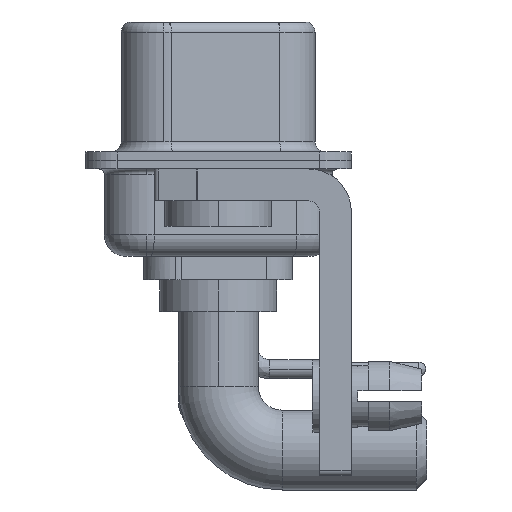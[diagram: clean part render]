
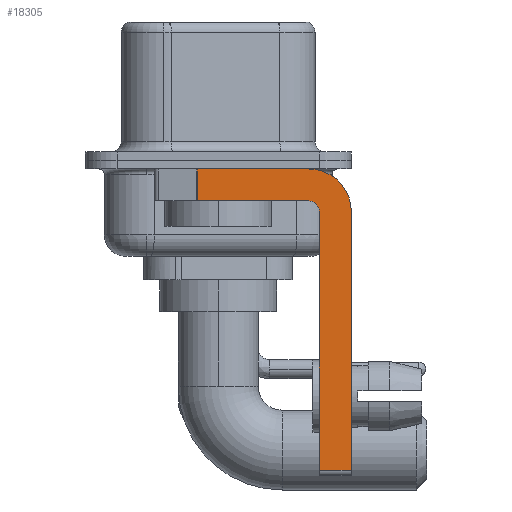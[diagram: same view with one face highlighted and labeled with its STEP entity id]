
A CAD part, left-side view. The second image highlights one B-rep face of the part: STEP entity #18305.
In plain terms, the highlighted planar face has unit normal (-1, 0, 0).
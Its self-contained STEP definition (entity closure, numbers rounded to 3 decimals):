
#687 = DIRECTION ( 'NONE',  ( 0., 0., 1. ) ) ;
#978 = CARTESIAN_POINT ( 'NONE',  ( -2.9, -4.25, -1.9 ) ) ;
#1161 = DIRECTION ( 'NONE',  ( 0., 0., -1. ) ) ;
#1473 = DIRECTION ( 'NONE',  ( 1., 0., 0. ) ) ;
#2070 = VERTEX_POINT ( 'NONE', #21945 ) ;
#2636 = CIRCLE ( 'NONE', #18275, 0.5 ) ;
#3033 = DIRECTION ( 'NONE',  ( 0., 0., 1. ) ) ;
#4359 = CARTESIAN_POINT ( 'NONE',  ( -2.9, -6.25, -2.4 ) ) ;
#4758 = VERTEX_POINT ( 'NONE', #16413 ) ;
#4934 = EDGE_CURVE ( 'NONE', #12364, #19871, #8243, .T. ) ;
#4981 = EDGE_LOOP ( 'NONE', ( #13253, #11088, #13358, #8289, #28068, #10919, #26692, #12249 ) ) ;
#5983 = CARTESIAN_POINT ( 'NONE',  ( -2.9, -4.25, -2.4 ) ) ;
#6004 = CARTESIAN_POINT ( 'NONE',  ( -2.9, -4.25, -1.9 ) ) ;
#7855 = EDGE_CURVE ( 'NONE', #4758, #14268, #2636, .T. ) ;
#7875 = CARTESIAN_POINT ( 'NONE',  ( -2.9, -4.25, -2.4 ) ) ;
#8243 = LINE ( 'NONE', #4359, #12987 ) ;
#8289 = ORIENTED_EDGE ( 'NONE', *, *, #7855, .F. ) ;
#8372 = DIRECTION ( 'NONE',  ( 1., 0., 0. ) ) ;
#8873 = CARTESIAN_POINT ( 'NONE',  ( -2.9, 3., -0.4 ) ) ;
#8938 = LINE ( 'NONE', #16047, #11588 ) ;
#10384 = VERTEX_POINT ( 'NONE', #18483 ) ;
#10616 = DIRECTION ( 'NONE',  ( 0., 0., -1. ) ) ;
#10919 = ORIENTED_EDGE ( 'NONE', *, *, #14473, .T. ) ;
#11088 = ORIENTED_EDGE ( 'NONE', *, *, #21189, .T. ) ;
#11556 = CARTESIAN_POINT ( 'NONE',  ( -2.9, -6.25, -14.55 ) ) ;
#11588 = VECTOR ( 'NONE', #25247, 1000. ) ;
#11960 = LINE ( 'NONE', #13356, #14738 ) ;
#12249 = ORIENTED_EDGE ( 'NONE', *, *, #23629, .F. ) ;
#12364 = VERTEX_POINT ( 'NONE', #16400 ) ;
#12987 = VECTOR ( 'NONE', #10616, 1000. ) ;
#13253 = ORIENTED_EDGE ( 'NONE', *, *, #22727, .F. ) ;
#13356 = CARTESIAN_POINT ( 'NONE',  ( -2.9, -4.75, -14.8 ) ) ;
#13358 = ORIENTED_EDGE ( 'NONE', *, *, #21850, .F. ) ;
#14268 = VERTEX_POINT ( 'NONE', #978 ) ;
#14317 = CARTESIAN_POINT ( 'NONE',  ( -2.9, -4.25, -2.4 ) ) ;
#14473 = EDGE_CURVE ( 'NONE', #2070, #19871, #8938, .T. ) ;
#14738 = VECTOR ( 'NONE', #687, 1000. ) ;
#14963 = EDGE_CURVE ( 'NONE', #2070, #4758, #11960, .T. ) ;
#14968 = CARTESIAN_POINT ( 'NONE',  ( -2.9, 0.978, -1.9 ) ) ;
#15361 = DIRECTION ( 'NONE',  ( 0., 1., 0. ) ) ;
#16047 = CARTESIAN_POINT ( 'NONE',  ( -2.9, -4.25, -14.55 ) ) ;
#16400 = CARTESIAN_POINT ( 'NONE',  ( -2.9, -6.25, -2.4 ) ) ;
#16413 = CARTESIAN_POINT ( 'NONE',  ( -2.9, -4.75, -2.4 ) ) ;
#16535 = CARTESIAN_POINT ( 'NONE',  ( -2.9, 0.978, -0.4 ) ) ;
#16927 = FACE_OUTER_BOUND ( 'NONE', #4981, .T. ) ;
#18275 = AXIS2_PLACEMENT_3D ( 'NONE', #14317, #21272, #3033 ) ;
#18305 = ADVANCED_FACE ( 'NONE', ( #16927 ), #28206, .F. ) ;
#18483 = CARTESIAN_POINT ( 'NONE',  ( -2.9, -4.25, -0.4 ) ) ;
#19671 = VECTOR ( 'NONE', #1161, 1000. ) ;
#19871 = VERTEX_POINT ( 'NONE', #11556 ) ;
#21189 = EDGE_CURVE ( 'NONE', #29241, #27691, #21487, .T. ) ;
#21272 = DIRECTION ( 'NONE',  ( -1., 0., 0. ) ) ;
#21487 = LINE ( 'NONE', #14968, #19671 ) ;
#21566 = VECTOR ( 'NONE', #15361, 1000. ) ;
#21850 = EDGE_CURVE ( 'NONE', #14268, #27691, #28855, .T. ) ;
#21945 = CARTESIAN_POINT ( 'NONE',  ( -2.9, -4.75, -14.55 ) ) ;
#21954 = DIRECTION ( 'NONE',  ( 0., 0., -1. ) ) ;
#22537 = AXIS2_PLACEMENT_3D ( 'NONE', #5983, #8372, #29128 ) ;
#22727 = EDGE_CURVE ( 'NONE', #29241, #10384, #29198, .T. ) ;
#23629 = EDGE_CURVE ( 'NONE', #10384, #12364, #24421, .T. ) ;
#24421 = CIRCLE ( 'NONE', #22537, 2. ) ;
#25247 = DIRECTION ( 'NONE',  ( 0., -1., 0. ) ) ;
#25819 = VECTOR ( 'NONE', #26669, 1000. ) ;
#26669 = DIRECTION ( 'NONE',  ( 0., -1., 0. ) ) ;
#26692 = ORIENTED_EDGE ( 'NONE', *, *, #4934, .F. ) ;
#27052 = AXIS2_PLACEMENT_3D ( 'NONE', #7875, #1473, #21954 ) ;
#27691 = VERTEX_POINT ( 'NONE', #28778 ) ;
#28068 = ORIENTED_EDGE ( 'NONE', *, *, #14963, .F. ) ;
#28206 = PLANE ( 'NONE',  #27052 ) ;
#28778 = CARTESIAN_POINT ( 'NONE',  ( -2.9, 0.978, -1.9 ) ) ;
#28855 = LINE ( 'NONE', #6004, #21566 ) ;
#29128 = DIRECTION ( 'NONE',  ( 0., 0., -1. ) ) ;
#29198 = LINE ( 'NONE', #8873, #25819 ) ;
#29241 = VERTEX_POINT ( 'NONE', #16535 ) ;
